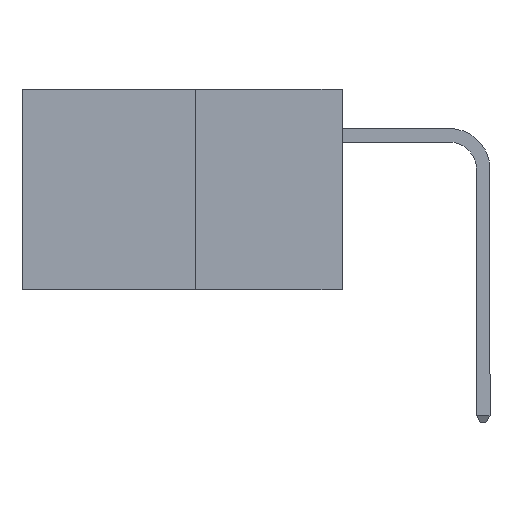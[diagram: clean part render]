
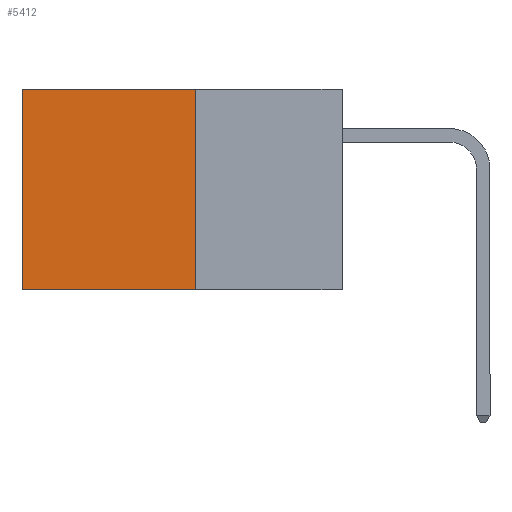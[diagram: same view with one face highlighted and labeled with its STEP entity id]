
A CAD part, left-side view. The second image highlights one B-rep face of the part: STEP entity #5412.
In plain terms, the highlighted planar face has unit normal (-1, 0, 0).
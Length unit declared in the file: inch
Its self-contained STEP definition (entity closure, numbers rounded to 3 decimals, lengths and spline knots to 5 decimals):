
#52 = DIRECTION ( 'NONE',  ( 0., 1., 0. ) ) ;
#113 = ORIENTED_EDGE ( 'NONE', *, *, #836, .F. ) ;
#527 = CARTESIAN_POINT ( 'NONE',  ( 0.277, 0.27, -0.37 ) ) ;
#759 = LINE ( 'NONE', #2806, #7318 ) ;
#836 = EDGE_CURVE ( 'NONE', #1690, #8411, #5551, .T. ) ;
#864 = CARTESIAN_POINT ( 'NONE',  ( 0.277, 0.59, -0.37 ) ) ;
#1481 = CARTESIAN_POINT ( 'NONE',  ( 0.277, 0.27, -0.37 ) ) ;
#1503 = VERTEX_POINT ( 'NONE', #2217 ) ;
#1690 = VERTEX_POINT ( 'NONE', #527 ) ;
#2217 = CARTESIAN_POINT ( 'NONE',  ( 0.277, 0.59, 0. ) ) ;
#2428 = PLANE ( 'NONE',  #5959 ) ;
#2431 = LINE ( 'NONE', #864, #7659 ) ;
#2486 = VERTEX_POINT ( 'NONE', #5952 ) ;
#2612 = DIRECTION ( 'NONE',  ( 0., 1., 0. ) ) ;
#2691 = DIRECTION ( 'NONE',  ( 0., 0., -1. ) ) ;
#2806 = CARTESIAN_POINT ( 'NONE',  ( 0.277, 0.27, 0. ) ) ;
#3296 = CARTESIAN_POINT ( 'NONE',  ( 0.277, 0.27, -0.37 ) ) ;
#3721 = EDGE_CURVE ( 'NONE', #2486, #1690, #7585, .T. ) ;
#3836 = VECTOR ( 'NONE', #52, 39.37008 ) ;
#4091 = CARTESIAN_POINT ( 'NONE',  ( 0.277, 0.27, -0.37 ) ) ;
#4791 = EDGE_CURVE ( 'NONE', #2486, #1503, #759, .T. ) ;
#4929 = CARTESIAN_POINT ( 'NONE',  ( 0.277, 0.59, -0.37 ) ) ;
#4975 = EDGE_LOOP ( 'NONE', ( #6857, #113, #6459, #6355 ) ) ;
#5204 = EDGE_CURVE ( 'NONE', #1503, #8411, #2431, .T. ) ;
#5412 = ADVANCED_FACE ( 'NONE', ( #7750 ), #2428, .F. ) ;
#5551 = LINE ( 'NONE', #4091, #3836 ) ;
#5790 = VECTOR ( 'NONE', #2691, 39.37008 ) ;
#5952 = CARTESIAN_POINT ( 'NONE',  ( 0.277, 0.27, 0. ) ) ;
#5959 = AXIS2_PLACEMENT_3D ( 'NONE', #3296, #7131, #8055 ) ;
#6345 = DIRECTION ( 'NONE',  ( 0., 0., -1. ) ) ;
#6355 = ORIENTED_EDGE ( 'NONE', *, *, #4791, .T. ) ;
#6459 = ORIENTED_EDGE ( 'NONE', *, *, #3721, .F. ) ;
#6857 = ORIENTED_EDGE ( 'NONE', *, *, #5204, .T. ) ;
#7131 = DIRECTION ( 'NONE',  ( 1., 0., 0. ) ) ;
#7318 = VECTOR ( 'NONE', #2612, 39.37008 ) ;
#7585 = LINE ( 'NONE', #1481, #5790 ) ;
#7659 = VECTOR ( 'NONE', #6345, 39.37008 ) ;
#7750 = FACE_OUTER_BOUND ( 'NONE', #4975, .T. ) ;
#8055 = DIRECTION ( 'NONE',  ( 0., 0., -1. ) ) ;
#8411 = VERTEX_POINT ( 'NONE', #4929 ) ;
